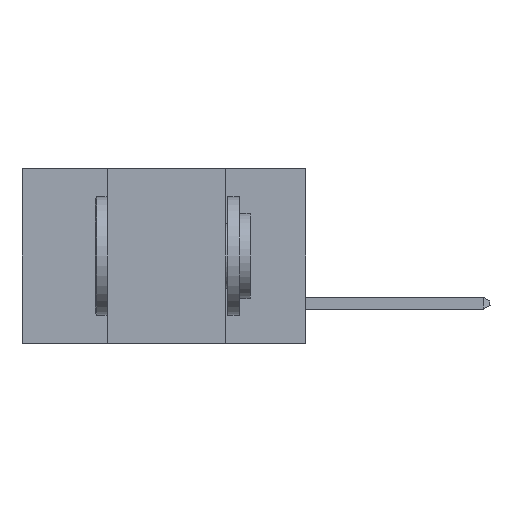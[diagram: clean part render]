
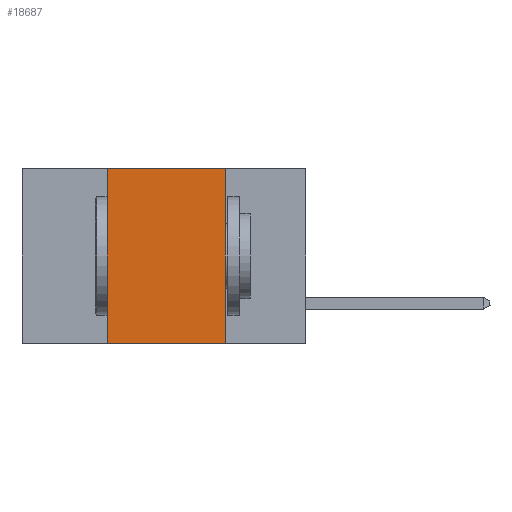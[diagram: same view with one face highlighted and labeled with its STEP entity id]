
A CAD part, left-side view. The second image highlights one B-rep face of the part: STEP entity #18687.
In plain terms, the highlighted planar face has unit normal (-1, 0, 0).
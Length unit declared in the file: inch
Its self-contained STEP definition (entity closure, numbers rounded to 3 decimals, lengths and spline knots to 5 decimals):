
#924 = VERTEX_POINT ( 'NONE', #1540 ) ;
#1506 = CARTESIAN_POINT ( 'NONE',  ( 0., 0.6, 0. ) ) ;
#1540 = CARTESIAN_POINT ( 'NONE',  ( 0., 0.17, 0. ) ) ;
#1663 = ORIENTED_EDGE ( 'NONE', *, *, #18063, .F. ) ;
#3097 = FACE_OUTER_BOUND ( 'NONE', #8308, .T. ) ;
#3169 = DIRECTION ( 'NONE',  ( 1., 0., 0. ) ) ;
#3914 = VECTOR ( 'NONE', #20356, 39.37008 ) ;
#5014 = PLANE ( 'NONE',  #11474 ) ;
#5047 = CARTESIAN_POINT ( 'NONE',  ( 0., 0.6, 0. ) ) ;
#5565 = CARTESIAN_POINT ( 'NONE',  ( 0., 0.42, -0.37 ) ) ;
#5752 = VERTEX_POINT ( 'NONE', #9602 ) ;
#6150 = VECTOR ( 'NONE', #13628, 39.37008 ) ;
#6964 = ORIENTED_EDGE ( 'NONE', *, *, #21618, .T. ) ;
#7916 = CARTESIAN_POINT ( 'NONE',  ( 0., 0.42, 0. ) ) ;
#7972 = CARTESIAN_POINT ( 'NONE',  ( 0., 0.17, 0. ) ) ;
#8308 = EDGE_LOOP ( 'NONE', ( #1663, #13893, #16548, #6964 ) ) ;
#8505 = LINE ( 'NONE', #7972, #3914 ) ;
#9602 = CARTESIAN_POINT ( 'NONE',  ( 0., 0.17, -0.37 ) ) ;
#9637 = VERTEX_POINT ( 'NONE', #7916 ) ;
#10148 = DIRECTION ( 'NONE',  ( 0., 0., -1. ) ) ;
#11191 = VECTOR ( 'NONE', #17418, 39.37008 ) ;
#11474 = AXIS2_PLACEMENT_3D ( 'NONE', #1506, #3169, #10148 ) ;
#12494 = CARTESIAN_POINT ( 'NONE',  ( 0., 0.42, 0. ) ) ;
#13628 = DIRECTION ( 'NONE',  ( 0., -1., 0. ) ) ;
#13893 = ORIENTED_EDGE ( 'NONE', *, *, #20881, .F. ) ;
#15578 = LINE ( 'NONE', #18408, #6150 ) ;
#15595 = VERTEX_POINT ( 'NONE', #5565 ) ;
#15745 = LINE ( 'NONE', #12494, #11191 ) ;
#16548 = ORIENTED_EDGE ( 'NONE', *, *, #18336, .F. ) ;
#17418 = DIRECTION ( 'NONE',  ( 0., 0., 1. ) ) ;
#17484 = VECTOR ( 'NONE', #20373, 39.37008 ) ;
#18063 = EDGE_CURVE ( 'NONE', #924, #5752, #8505, .T. ) ;
#18336 = EDGE_CURVE ( 'NONE', #15595, #9637, #15745, .T. ) ;
#18408 = CARTESIAN_POINT ( 'NONE',  ( 0., 0.6, -0.37 ) ) ;
#18687 = ADVANCED_FACE ( 'NONE', ( #3097 ), #5014, .F. ) ;
#20179 = LINE ( 'NONE', #5047, #17484 ) ;
#20356 = DIRECTION ( 'NONE',  ( 0., 0., -1. ) ) ;
#20373 = DIRECTION ( 'NONE',  ( 0., -1., 0. ) ) ;
#20881 = EDGE_CURVE ( 'NONE', #9637, #924, #20179, .T. ) ;
#21618 = EDGE_CURVE ( 'NONE', #15595, #5752, #15578, .T. ) ;
